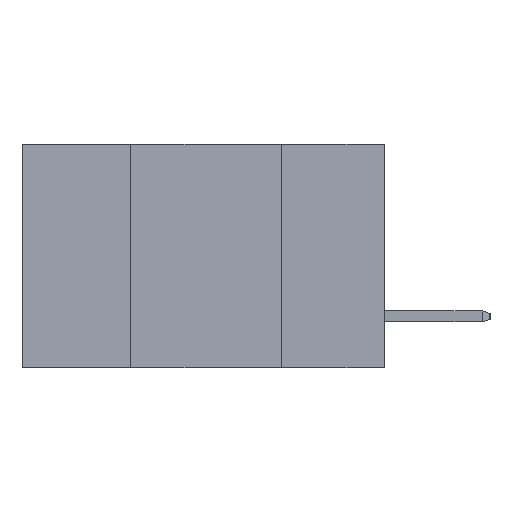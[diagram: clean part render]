
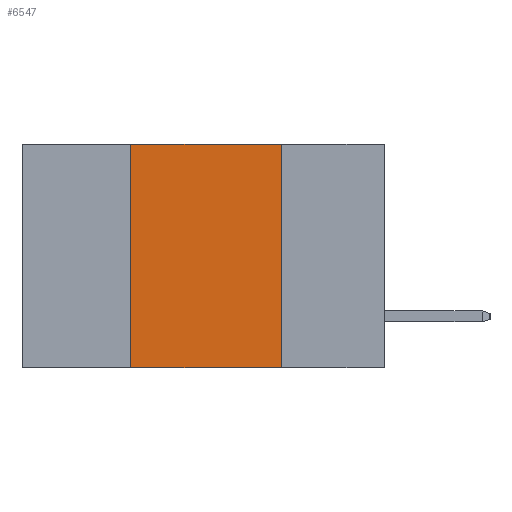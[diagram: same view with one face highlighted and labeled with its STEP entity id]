
A CAD part, left-side view. The second image highlights one B-rep face of the part: STEP entity #6547.
In plain terms, the highlighted planar face has unit normal (-1, 0, 0).
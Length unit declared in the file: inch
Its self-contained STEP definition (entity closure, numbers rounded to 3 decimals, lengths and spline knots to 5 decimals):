
#681 = VECTOR ( 'NONE', #5387, 39.37008 ) ;
#739 = CARTESIAN_POINT ( 'NONE',  ( 0., 0.17, 0. ) ) ;
#827 = CARTESIAN_POINT ( 'NONE',  ( 0., 0.42, -0.37 ) ) ;
#890 = EDGE_CURVE ( 'NONE', #8613, #3900, #1366, .T. ) ;
#1163 = VECTOR ( 'NONE', #5855, 39.37008 ) ;
#1366 = LINE ( 'NONE', #5666, #10232 ) ;
#1401 = ORIENTED_EDGE ( 'NONE', *, *, #890, .T. ) ;
#2345 = DIRECTION ( 'NONE',  ( 0., 0., 1. ) ) ;
#2676 = CARTESIAN_POINT ( 'NONE',  ( 0., 0.42, 0. ) ) ;
#2825 = CARTESIAN_POINT ( 'NONE',  ( 0., 0.6, 0. ) ) ;
#3900 = VERTEX_POINT ( 'NONE', #8280 ) ;
#4038 = ORIENTED_EDGE ( 'NONE', *, *, #4556, .F. ) ;
#4090 = CARTESIAN_POINT ( 'NONE',  ( 0., 0.42, 0. ) ) ;
#4556 = EDGE_CURVE ( 'NONE', #5588, #9921, #6442, .T. ) ;
#5185 = AXIS2_PLACEMENT_3D ( 'NONE', #2825, #10299, #10289 ) ;
#5387 = DIRECTION ( 'NONE',  ( 0., 0., -1. ) ) ;
#5588 = VERTEX_POINT ( 'NONE', #2676 ) ;
#5666 = CARTESIAN_POINT ( 'NONE',  ( 0., 0.6, -0.37 ) ) ;
#5800 = DIRECTION ( 'NONE',  ( 0., -1., 0. ) ) ;
#5855 = DIRECTION ( 'NONE',  ( 0., -1., 0. ) ) ;
#6282 = CARTESIAN_POINT ( 'NONE',  ( 0., 0.17, 0. ) ) ;
#6442 = LINE ( 'NONE', #8462, #1163 ) ;
#6547 = ADVANCED_FACE ( 'NONE', ( #8907 ), #8350, .F. ) ;
#7730 = LINE ( 'NONE', #6282, #681 ) ;
#8280 = CARTESIAN_POINT ( 'NONE',  ( 0., 0.17, -0.37 ) ) ;
#8350 = PLANE ( 'NONE',  #5185 ) ;
#8369 = VECTOR ( 'NONE', #2345, 39.37008 ) ;
#8462 = CARTESIAN_POINT ( 'NONE',  ( 0., 0.6, 0. ) ) ;
#8613 = VERTEX_POINT ( 'NONE', #827 ) ;
#8653 = ORIENTED_EDGE ( 'NONE', *, *, #8734, .F. ) ;
#8734 = EDGE_CURVE ( 'NONE', #9921, #3900, #7730, .T. ) ;
#8907 = FACE_OUTER_BOUND ( 'NONE', #10534, .T. ) ;
#9271 = EDGE_CURVE ( 'NONE', #8613, #5588, #10486, .T. ) ;
#9921 = VERTEX_POINT ( 'NONE', #739 ) ;
#10232 = VECTOR ( 'NONE', #5800, 39.37008 ) ;
#10289 = DIRECTION ( 'NONE',  ( 0., 0., -1. ) ) ;
#10299 = DIRECTION ( 'NONE',  ( 1., 0., 0. ) ) ;
#10486 = LINE ( 'NONE', #4090, #8369 ) ;
#10527 = ORIENTED_EDGE ( 'NONE', *, *, #9271, .F. ) ;
#10534 = EDGE_LOOP ( 'NONE', ( #8653, #4038, #10527, #1401 ) ) ;
